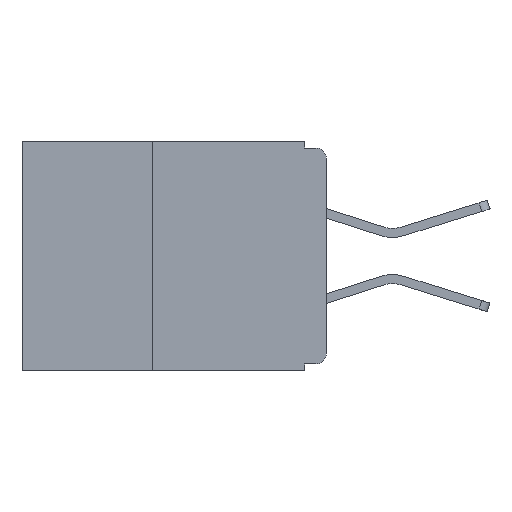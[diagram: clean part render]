
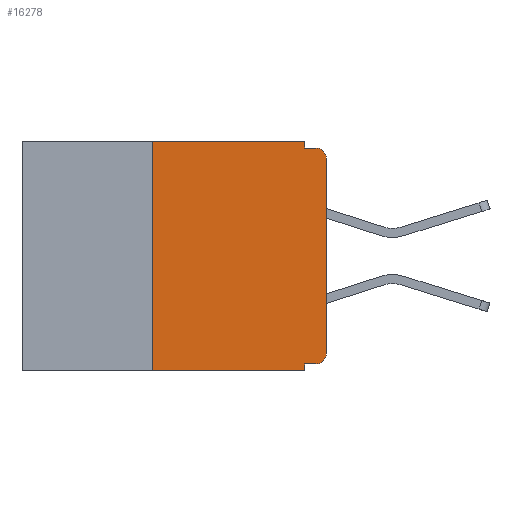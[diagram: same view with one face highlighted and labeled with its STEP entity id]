
A CAD part, left-side view. The second image highlights one B-rep face of the part: STEP entity #16278.
In plain terms, the highlighted planar face has unit normal (-1, 0, 0).
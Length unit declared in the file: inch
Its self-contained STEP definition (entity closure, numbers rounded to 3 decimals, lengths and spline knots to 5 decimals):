
#162 = CARTESIAN_POINT ( 'NONE',  ( 0., 0.031, 0. ) ) ;
#970 = ORIENTED_EDGE ( 'NONE', *, *, #21577, .T. ) ;
#1244 = ORIENTED_EDGE ( 'NONE', *, *, #15468, .F. ) ;
#1616 = DIRECTION ( 'NONE',  ( -1., 0., 0. ) ) ;
#1873 = ORIENTED_EDGE ( 'NONE', *, *, #18200, .F. ) ;
#2090 = ORIENTED_EDGE ( 'NONE', *, *, #29942, .F. ) ;
#2811 = EDGE_CURVE ( 'NONE', #27843, #4677, #6978, .T. ) ;
#3738 = AXIS2_PLACEMENT_3D ( 'NONE', #16449, #1616, #18898 ) ;
#3786 = AXIS2_PLACEMENT_3D ( 'NONE', #22577, #7871, #24980 ) ;
#3944 = ORIENTED_EDGE ( 'NONE', *, *, #9975, .F. ) ;
#4069 = ORIENTED_EDGE ( 'NONE', *, *, #8341, .T. ) ;
#4209 = VERTEX_POINT ( 'NONE', #24523 ) ;
#4677 = VERTEX_POINT ( 'NONE', #13938 ) ;
#4725 = LINE ( 'NONE', #7827, #12077 ) ;
#4732 = CARTESIAN_POINT ( 'NONE',  ( 0., 0., -0.305 ) ) ;
#4738 = VERTEX_POINT ( 'NONE', #6686 ) ;
#5674 = ORIENTED_EDGE ( 'NONE', *, *, #8484, .F. ) ;
#5782 = CARTESIAN_POINT ( 'NONE',  ( 0., 0.437, 0. ) ) ;
#5926 = ORIENTED_EDGE ( 'NONE', *, *, #2811, .F. ) ;
#6686 = CARTESIAN_POINT ( 'NONE',  ( 0., 0.031, -0.01 ) ) ;
#6978 = LINE ( 'NONE', #28378, #12819 ) ;
#7651 = ORIENTED_EDGE ( 'NONE', *, *, #23817, .T. ) ;
#7827 = CARTESIAN_POINT ( 'NONE',  ( 0., 0., -0.01 ) ) ;
#7871 = DIRECTION ( 'NONE',  ( -1., 0., 0. ) ) ;
#8341 = EDGE_CURVE ( 'NONE', #19840, #22585, #22368, .T. ) ;
#8484 = EDGE_CURVE ( 'NONE', #4677, #22585, #18512, .T. ) ;
#9334 = DIRECTION ( 'NONE',  ( 0., 0., 1. ) ) ;
#9501 = CARTESIAN_POINT ( 'NONE',  ( 0., 0.031, -0.33 ) ) ;
#9949 = FACE_OUTER_BOUND ( 'NONE', #13712, .T. ) ;
#9975 = EDGE_CURVE ( 'NONE', #19840, #19678, #27999, .T. ) ;
#10150 = DIRECTION ( 'NONE',  ( 0., 0., -1. ) ) ;
#10575 = VERTEX_POINT ( 'NONE', #18934 ) ;
#10996 = VECTOR ( 'NONE', #22984, 39.37008 ) ;
#11394 = LINE ( 'NONE', #162, #23657 ) ;
#11534 = PLANE ( 'NONE',  #19167 ) ;
#11976 = DIRECTION ( 'NONE',  ( 0., 0., -1. ) ) ;
#12077 = VECTOR ( 'NONE', #22533, 39.37008 ) ;
#12213 = VERTEX_POINT ( 'NONE', #12361 ) ;
#12361 = CARTESIAN_POINT ( 'NONE',  ( 0., 0.015, -0.01 ) ) ;
#12819 = VECTOR ( 'NONE', #28268, 39.37008 ) ;
#13311 = CARTESIAN_POINT ( 'NONE',  ( 0., 0.031, -0.33 ) ) ;
#13475 = CARTESIAN_POINT ( 'NONE',  ( 0., 0., 0. ) ) ;
#13712 = EDGE_LOOP ( 'NONE', ( #31358, #970, #1244, #1873, #2090, #3944, #4069, #5674, #5926, #7651 ) ) ;
#13938 = CARTESIAN_POINT ( 'NONE',  ( 0., 0.031, -0.32 ) ) ;
#14020 = DIRECTION ( 'NONE',  ( 0., 0., -1. ) ) ;
#15468 = EDGE_CURVE ( 'NONE', #4738, #12213, #4725, .T. ) ;
#15853 = CARTESIAN_POINT ( 'NONE',  ( 0., 0.437, -0.33 ) ) ;
#16278 = ADVANCED_FACE ( 'NONE', ( #9949 ), #11534, .F. ) ;
#16449 = CARTESIAN_POINT ( 'NONE',  ( 0., 0.015, -0.025 ) ) ;
#16631 = CARTESIAN_POINT ( 'NONE',  ( 0., 0.25, -0.33 ) ) ;
#17384 = VECTOR ( 'NONE', #30369, 39.37008 ) ;
#18111 = CARTESIAN_POINT ( 'NONE',  ( 0., 0.25, 0. ) ) ;
#18200 = EDGE_CURVE ( 'NONE', #4209, #4738, #11394, .T. ) ;
#18512 = LINE ( 'NONE', #9501, #31354 ) ;
#18898 = DIRECTION ( 'NONE',  ( 0., 0., -1. ) ) ;
#18934 = CARTESIAN_POINT ( 'NONE',  ( 0., 0., -0.025 ) ) ;
#19167 = AXIS2_PLACEMENT_3D ( 'NONE', #23743, #28565, #14020 ) ;
#19678 = VERTEX_POINT ( 'NONE', #18111 ) ;
#19840 = VERTEX_POINT ( 'NONE', #23542 ) ;
#21092 = VERTEX_POINT ( 'NONE', #4732 ) ;
#21577 = EDGE_CURVE ( 'NONE', #10575, #12213, #30212, .T. ) ;
#21589 = VECTOR ( 'NONE', #9334, 39.37008 ) ;
#22215 = CIRCLE ( 'NONE', #3786, 0.015 ) ;
#22368 = LINE ( 'NONE', #15853, #17384 ) ;
#22518 = LINE ( 'NONE', #5782, #10996 ) ;
#22533 = DIRECTION ( 'NONE',  ( 0., -1., 0. ) ) ;
#22577 = CARTESIAN_POINT ( 'NONE',  ( 0., 0.015, -0.305 ) ) ;
#22585 = VERTEX_POINT ( 'NONE', #13311 ) ;
#22984 = DIRECTION ( 'NONE',  ( 0., -1., 0. ) ) ;
#23542 = CARTESIAN_POINT ( 'NONE',  ( 0., 0.25, -0.33 ) ) ;
#23657 = VECTOR ( 'NONE', #10150, 39.37008 ) ;
#23743 = CARTESIAN_POINT ( 'NONE',  ( 0., 0.437, 0. ) ) ;
#23817 = EDGE_CURVE ( 'NONE', #27843, #21092, #22215, .T. ) ;
#24365 = LINE ( 'NONE', #13475, #29260 ) ;
#24523 = CARTESIAN_POINT ( 'NONE',  ( 0., 0.031, 0. ) ) ;
#24980 = DIRECTION ( 'NONE',  ( 0., 0., -1. ) ) ;
#25602 = DIRECTION ( 'NONE',  ( 0., 0., 1. ) ) ;
#25804 = CARTESIAN_POINT ( 'NONE',  ( 0., 0.015, -0.32 ) ) ;
#27843 = VERTEX_POINT ( 'NONE', #25804 ) ;
#27999 = LINE ( 'NONE', #16631, #21589 ) ;
#28268 = DIRECTION ( 'NONE',  ( 0., 1., 0. ) ) ;
#28378 = CARTESIAN_POINT ( 'NONE',  ( 0., 0., -0.32 ) ) ;
#28565 = DIRECTION ( 'NONE',  ( 1., 0., 0. ) ) ;
#29260 = VECTOR ( 'NONE', #25602, 39.37008 ) ;
#29481 = EDGE_CURVE ( 'NONE', #21092, #10575, #24365, .T. ) ;
#29942 = EDGE_CURVE ( 'NONE', #19678, #4209, #22518, .T. ) ;
#30212 = CIRCLE ( 'NONE', #3738, 0.015 ) ;
#30369 = DIRECTION ( 'NONE',  ( 0., -1., 0. ) ) ;
#31354 = VECTOR ( 'NONE', #11976, 39.37008 ) ;
#31358 = ORIENTED_EDGE ( 'NONE', *, *, #29481, .T. ) ;
